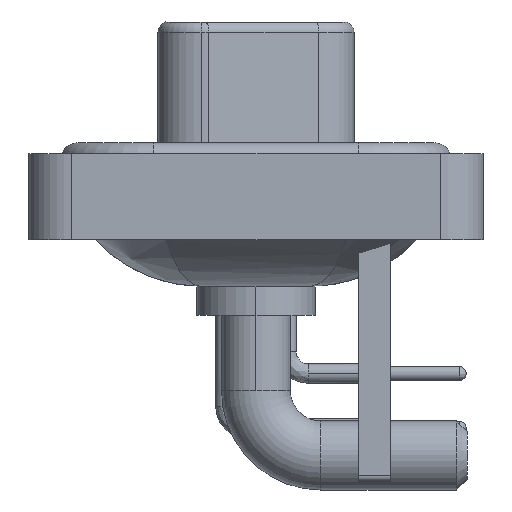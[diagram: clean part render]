
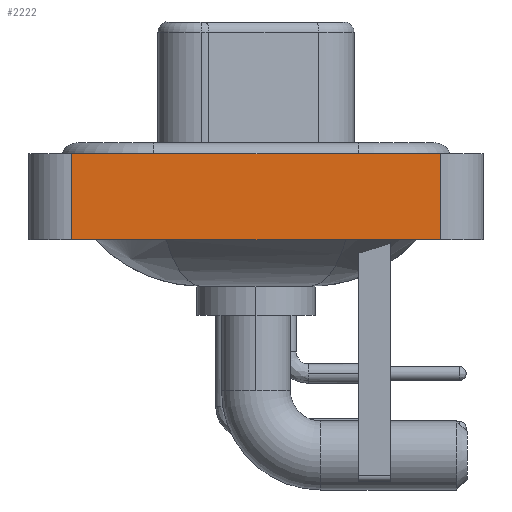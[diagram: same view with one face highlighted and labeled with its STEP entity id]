
A CAD part, left-side view. The second image highlights one B-rep face of the part: STEP entity #2222.
In plain terms, the highlighted planar face has unit normal (-1, 0, 0).
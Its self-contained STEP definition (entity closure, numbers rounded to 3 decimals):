
#1703 = CARTESIAN_POINT ( 'NONE',  ( -7.3, -8.55, 0.4 ) ) ;
#2222 = ADVANCED_FACE ( 'NONE', ( #2264 ), #18373, .T. ) ;
#2264 = FACE_OUTER_BOUND ( 'NONE', #16941, .T. ) ;
#4307 = VECTOR ( 'NONE', #19426, 1000. ) ;
#4579 = ORIENTED_EDGE ( 'NONE', *, *, #10399, .F. ) ;
#5849 = CARTESIAN_POINT ( 'NONE',  ( -7.3, 8.55, -3.6 ) ) ;
#6427 = DIRECTION ( 'NONE',  ( 0., 0., 1. ) ) ;
#6625 = EDGE_CURVE ( 'NONE', #9524, #13133, #8229, .T. ) ;
#7520 = LINE ( 'NONE', #7638, #13775 ) ;
#7638 = CARTESIAN_POINT ( 'NONE',  ( -7.3, -8.55, -3.6 ) ) ;
#8229 = LINE ( 'NONE', #16050, #21519 ) ;
#8656 = EDGE_CURVE ( 'NONE', #14820, #9524, #7520, .T. ) ;
#9494 = DIRECTION ( 'NONE',  ( 0., -1., 0. ) ) ;
#9524 = VERTEX_POINT ( 'NONE', #13278 ) ;
#10399 = EDGE_CURVE ( 'NONE', #14820, #10675, #21611, .T. ) ;
#10442 = ORIENTED_EDGE ( 'NONE', *, *, #17499, .F. ) ;
#10675 = VERTEX_POINT ( 'NONE', #22754 ) ;
#12233 = CARTESIAN_POINT ( 'NONE',  ( -7.3, -8.55, -3.6 ) ) ;
#12524 = ORIENTED_EDGE ( 'NONE', *, *, #8656, .T. ) ;
#13133 = VERTEX_POINT ( 'NONE', #18657 ) ;
#13278 = CARTESIAN_POINT ( 'NONE',  ( -7.3, -8.55, -3.6 ) ) ;
#13775 = VECTOR ( 'NONE', #15479, 1000. ) ;
#14281 = DIRECTION ( 'NONE',  ( -1., 0., 0. ) ) ;
#14351 = AXIS2_PLACEMENT_3D ( 'NONE', #12233, #14281, #22083 ) ;
#14379 = ORIENTED_EDGE ( 'NONE', *, *, #6625, .T. ) ;
#14820 = VERTEX_POINT ( 'NONE', #24885 ) ;
#15479 = DIRECTION ( 'NONE',  ( 0., -1., 0. ) ) ;
#16050 = CARTESIAN_POINT ( 'NONE',  ( -7.3, -8.55, -3.6 ) ) ;
#16898 = VECTOR ( 'NONE', #9494, 1000. ) ;
#16941 = EDGE_LOOP ( 'NONE', ( #14379, #10442, #4579, #12524 ) ) ;
#17499 = EDGE_CURVE ( 'NONE', #10675, #13133, #19217, .T. ) ;
#18373 = PLANE ( 'NONE',  #14351 ) ;
#18657 = CARTESIAN_POINT ( 'NONE',  ( -7.3, -8.55, 0.4 ) ) ;
#19217 = LINE ( 'NONE', #1703, #16898 ) ;
#19426 = DIRECTION ( 'NONE',  ( 0., 0., 1. ) ) ;
#21519 = VECTOR ( 'NONE', #6427, 1000. ) ;
#21611 = LINE ( 'NONE', #5849, #4307 ) ;
#22083 = DIRECTION ( 'NONE',  ( 0., 0., 1. ) ) ;
#22754 = CARTESIAN_POINT ( 'NONE',  ( -7.3, 8.55, 0.4 ) ) ;
#24885 = CARTESIAN_POINT ( 'NONE',  ( -7.3, 8.55, -3.6 ) ) ;
